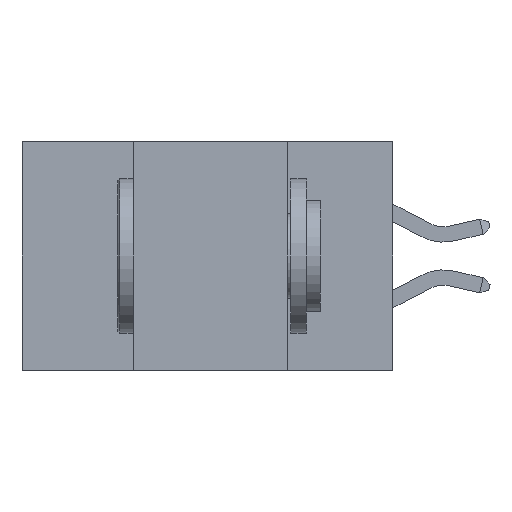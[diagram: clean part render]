
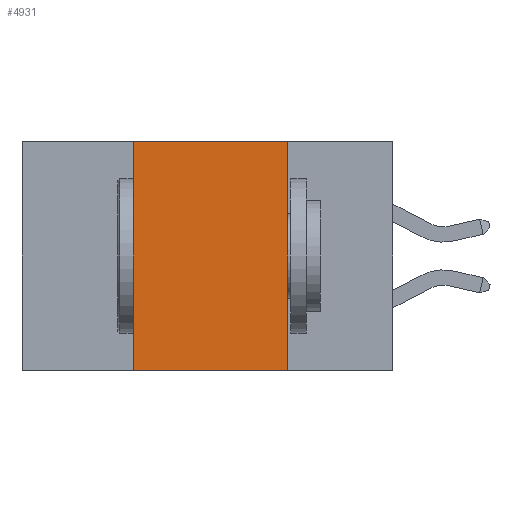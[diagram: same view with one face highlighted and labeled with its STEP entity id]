
A CAD part, left-side view. The second image highlights one B-rep face of the part: STEP entity #4931.
In plain terms, the highlighted planar face has unit normal (-1, 0, 0).
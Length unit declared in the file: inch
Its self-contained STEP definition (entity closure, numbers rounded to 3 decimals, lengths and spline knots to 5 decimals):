
#41 = CARTESIAN_POINT ( 'NONE',  ( 0., 0.6, -0.37 ) ) ;
#1186 = EDGE_CURVE ( 'NONE', #1894, #3396, #1818, .T. ) ;
#1496 = LINE ( 'NONE', #41, #5719 ) ;
#1782 = LINE ( 'NONE', #9274, #6122 ) ;
#1818 = LINE ( 'NONE', #5900, #3719 ) ;
#1878 = CARTESIAN_POINT ( 'NONE',  ( 0., 0.6, 0. ) ) ;
#1894 = VERTEX_POINT ( 'NONE', #5747 ) ;
#2180 = DIRECTION ( 'NONE',  ( 0., -1., 0. ) ) ;
#3396 = VERTEX_POINT ( 'NONE', #5078 ) ;
#3719 = VECTOR ( 'NONE', #2180, 39.37008 ) ;
#3850 = FACE_OUTER_BOUND ( 'NONE', #7879, .T. ) ;
#4047 = DIRECTION ( 'NONE',  ( 0., 0., 1. ) ) ;
#4153 = VERTEX_POINT ( 'NONE', #8404 ) ;
#4735 = CARTESIAN_POINT ( 'NONE',  ( 0., 0.17, 0. ) ) ;
#4797 = ORIENTED_EDGE ( 'NONE', *, *, #7462, .F. ) ;
#4931 = ADVANCED_FACE ( 'NONE', ( #3850 ), #8772, .F. ) ;
#5078 = CARTESIAN_POINT ( 'NONE',  ( 0., 0.17, 0. ) ) ;
#5380 = VERTEX_POINT ( 'NONE', #7157 ) ;
#5719 = VECTOR ( 'NONE', #8604, 39.37008 ) ;
#5747 = CARTESIAN_POINT ( 'NONE',  ( 0., 0.42, 0. ) ) ;
#5855 = VECTOR ( 'NONE', #6397, 39.37008 ) ;
#5900 = CARTESIAN_POINT ( 'NONE',  ( 0., 0.6, 0. ) ) ;
#6122 = VECTOR ( 'NONE', #4047, 39.37008 ) ;
#6128 = ORIENTED_EDGE ( 'NONE', *, *, #7622, .T. ) ;
#6397 = DIRECTION ( 'NONE',  ( 0., 0., -1. ) ) ;
#6788 = LINE ( 'NONE', #4735, #5855 ) ;
#7030 = AXIS2_PLACEMENT_3D ( 'NONE', #1878, #7913, #10530 ) ;
#7157 = CARTESIAN_POINT ( 'NONE',  ( 0., 0.17, -0.37 ) ) ;
#7462 = EDGE_CURVE ( 'NONE', #4153, #1894, #1782, .T. ) ;
#7622 = EDGE_CURVE ( 'NONE', #4153, #5380, #1496, .T. ) ;
#7879 = EDGE_LOOP ( 'NONE', ( #10592, #9623, #4797, #6128 ) ) ;
#7913 = DIRECTION ( 'NONE',  ( 1., 0., 0. ) ) ;
#8404 = CARTESIAN_POINT ( 'NONE',  ( 0., 0.42, -0.37 ) ) ;
#8604 = DIRECTION ( 'NONE',  ( 0., -1., 0. ) ) ;
#8772 = PLANE ( 'NONE',  #7030 ) ;
#9274 = CARTESIAN_POINT ( 'NONE',  ( 0., 0.42, 0. ) ) ;
#9623 = ORIENTED_EDGE ( 'NONE', *, *, #1186, .F. ) ;
#10530 = DIRECTION ( 'NONE',  ( 0., 0., -1. ) ) ;
#10592 = ORIENTED_EDGE ( 'NONE', *, *, #10629, .F. ) ;
#10629 = EDGE_CURVE ( 'NONE', #3396, #5380, #6788, .T. ) ;
